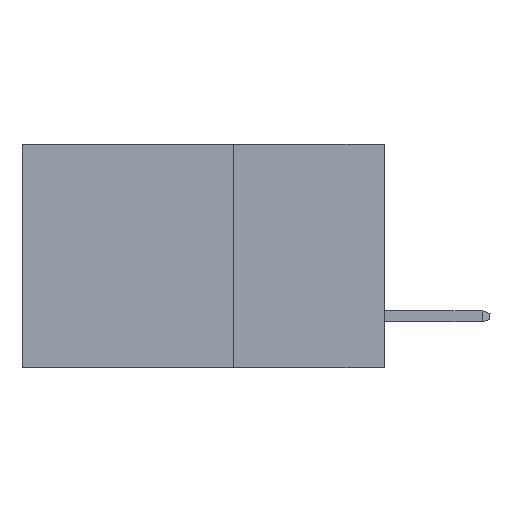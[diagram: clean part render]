
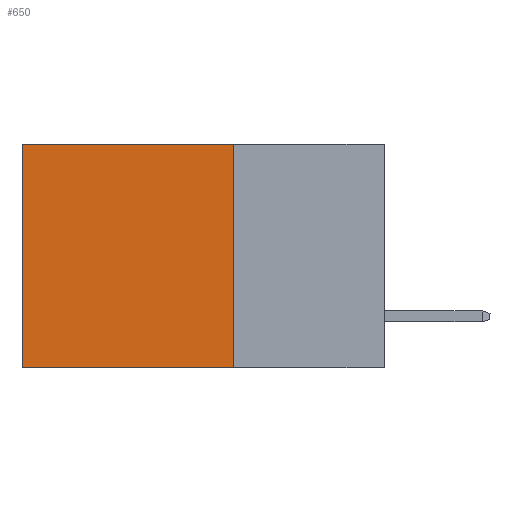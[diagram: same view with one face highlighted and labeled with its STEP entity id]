
A CAD part, left-side view. The second image highlights one B-rep face of the part: STEP entity #650.
In plain terms, the highlighted planar face has unit normal (-1, 0, 0).
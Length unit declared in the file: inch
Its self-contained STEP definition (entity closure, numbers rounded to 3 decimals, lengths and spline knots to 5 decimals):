
#33 = CARTESIAN_POINT ( 'NONE',  ( 0.2615, 0.25, -0.37 ) ) ;
#159 = EDGE_CURVE ( 'NONE', #7438, #3494, #3670, .T. ) ;
#550 = DIRECTION ( 'NONE',  ( 0., 1., 0. ) ) ;
#650 = ADVANCED_FACE ( 'NONE', ( #3132 ), #7791, .F. ) ;
#1131 = EDGE_CURVE ( 'NONE', #7957, #7438, #2570, .T. ) ;
#1242 = VECTOR ( 'NONE', #550, 39.37008 ) ;
#1264 = EDGE_CURVE ( 'NONE', #7957, #4191, #4014, .T. ) ;
#1481 = ORIENTED_EDGE ( 'NONE', *, *, #1264, .F. ) ;
#1752 = ORIENTED_EDGE ( 'NONE', *, *, #6627, .F. ) ;
#1843 = AXIS2_PLACEMENT_3D ( 'NONE', #4257, #3897, #8347 ) ;
#2368 = ORIENTED_EDGE ( 'NONE', *, *, #159, .T. ) ;
#2391 = ORIENTED_EDGE ( 'NONE', *, *, #1131, .T. ) ;
#2570 = LINE ( 'NONE', #7096, #4357 ) ;
#3132 = FACE_OUTER_BOUND ( 'NONE', #7310, .T. ) ;
#3358 = VECTOR ( 'NONE', #3751, 39.37008 ) ;
#3494 = VERTEX_POINT ( 'NONE', #3744 ) ;
#3670 = LINE ( 'NONE', #7553, #3358 ) ;
#3744 = CARTESIAN_POINT ( 'NONE',  ( 0.2615, 0.6, -0.37 ) ) ;
#3751 = DIRECTION ( 'NONE',  ( 0., 0., -1. ) ) ;
#3897 = DIRECTION ( 'NONE',  ( 1., 0., 0. ) ) ;
#3933 = DIRECTION ( 'NONE',  ( 0., 0., -1. ) ) ;
#4014 = LINE ( 'NONE', #33, #6524 ) ;
#4191 = VERTEX_POINT ( 'NONE', #4739 ) ;
#4257 = CARTESIAN_POINT ( 'NONE',  ( 0.2615, 0.25, -0.37 ) ) ;
#4357 = VECTOR ( 'NONE', #7133, 39.37008 ) ;
#4739 = CARTESIAN_POINT ( 'NONE',  ( 0.2615, 0.25, -0.37 ) ) ;
#6425 = CARTESIAN_POINT ( 'NONE',  ( 0.2615, 0.6, 0. ) ) ;
#6524 = VECTOR ( 'NONE', #3933, 39.37008 ) ;
#6627 = EDGE_CURVE ( 'NONE', #4191, #3494, #8300, .T. ) ;
#7096 = CARTESIAN_POINT ( 'NONE',  ( 0.2615, 0.25, 0. ) ) ;
#7133 = DIRECTION ( 'NONE',  ( 0., 1., 0. ) ) ;
#7310 = EDGE_LOOP ( 'NONE', ( #2368, #1752, #1481, #2391 ) ) ;
#7438 = VERTEX_POINT ( 'NONE', #6425 ) ;
#7553 = CARTESIAN_POINT ( 'NONE',  ( 0.2615, 0.6, -0.37 ) ) ;
#7703 = CARTESIAN_POINT ( 'NONE',  ( 0.2615, 0.25, -0.37 ) ) ;
#7791 = PLANE ( 'NONE',  #1843 ) ;
#7921 = CARTESIAN_POINT ( 'NONE',  ( 0.2615, 0.25, 0. ) ) ;
#7957 = VERTEX_POINT ( 'NONE', #7921 ) ;
#8300 = LINE ( 'NONE', #7703, #1242 ) ;
#8347 = DIRECTION ( 'NONE',  ( 0., 0., -1. ) ) ;
